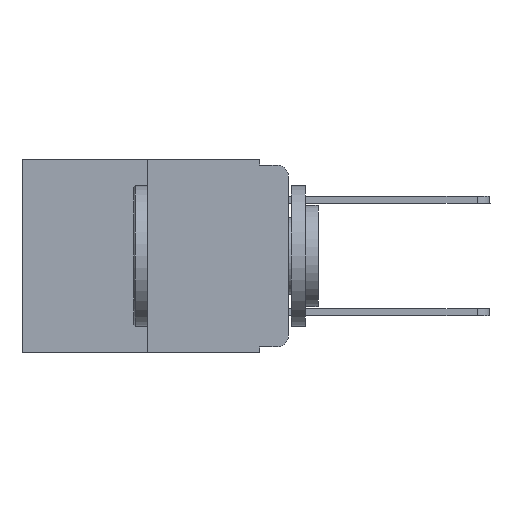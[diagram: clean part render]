
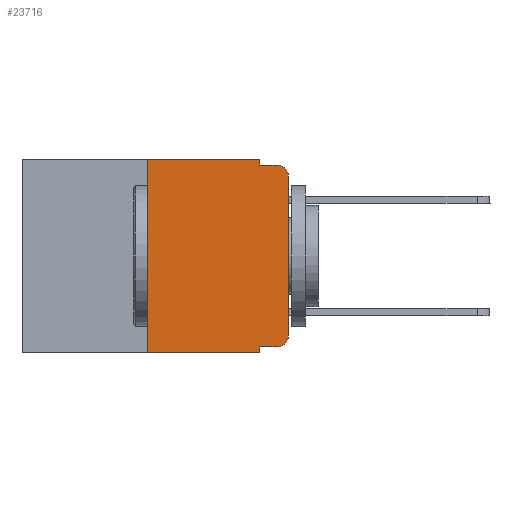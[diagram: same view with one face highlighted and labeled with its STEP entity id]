
A CAD part, left-side view. The second image highlights one B-rep face of the part: STEP entity #23716.
In plain terms, the highlighted planar face has unit normal (-1, 0, 0).
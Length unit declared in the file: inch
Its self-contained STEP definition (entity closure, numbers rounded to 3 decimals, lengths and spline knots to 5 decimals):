
#89 = DIRECTION ( 'NONE',  ( 0., 0., -1. ) ) ;
#220 = ORIENTED_EDGE ( 'NONE', *, *, #4690, .F. ) ;
#680 = CIRCLE ( 'NONE', #20054, 0.02 ) ;
#871 = VERTEX_POINT ( 'NONE', #3293 ) ;
#924 = AXIS2_PLACEMENT_3D ( 'NONE', #10022, #13965, #18078 ) ;
#1179 = ORIENTED_EDGE ( 'NONE', *, *, #4144, .T. ) ;
#1910 = ORIENTED_EDGE ( 'NONE', *, *, #21762, .T. ) ;
#2363 = VERTEX_POINT ( 'NONE', #22187 ) ;
#2385 = VECTOR ( 'NONE', #25052, 39.37008 ) ;
#2417 = CARTESIAN_POINT ( 'NONE',  ( 0., 0.051, -0.01 ) ) ;
#2907 = VERTEX_POINT ( 'NONE', #18002 ) ;
#3293 = CARTESIAN_POINT ( 'NONE',  ( 0., 0.051, -0.343 ) ) ;
#3735 = VECTOR ( 'NONE', #11981, 39.37008 ) ;
#3877 = VECTOR ( 'NONE', #17436, 39.37008 ) ;
#4144 = EDGE_CURVE ( 'NONE', #19177, #871, #5651, .T. ) ;
#4202 = VECTOR ( 'NONE', #18086, 39.37008 ) ;
#4552 = AXIS2_PLACEMENT_3D ( 'NONE', #26054, #11667, #21671 ) ;
#4689 = CARTESIAN_POINT ( 'NONE',  ( 0., 0.02, -0.333 ) ) ;
#4690 = EDGE_CURVE ( 'NONE', #19177, #2363, #14123, .T. ) ;
#4944 = CARTESIAN_POINT ( 'NONE',  ( 0., 0.051, 0. ) ) ;
#5037 = EDGE_CURVE ( 'NONE', #26030, #22423, #17229, .T. ) ;
#5310 = EDGE_CURVE ( 'NONE', #17140, #22423, #14396, .T. ) ;
#5575 = LINE ( 'NONE', #4944, #2385 ) ;
#5651 = LINE ( 'NONE', #24062, #3735 ) ;
#5678 = CARTESIAN_POINT ( 'NONE',  ( 0., 0.051, -0.333 ) ) ;
#5713 = EDGE_CURVE ( 'NONE', #19248, #26030, #5575, .T. ) ;
#6351 = FACE_OUTER_BOUND ( 'NONE', #14329, .T. ) ;
#6601 = ORIENTED_EDGE ( 'NONE', *, *, #5037, .F. ) ;
#8205 = CARTESIAN_POINT ( 'NONE',  ( 0., 0.02, -0.313 ) ) ;
#9725 = VECTOR ( 'NONE', #14063, 39.37008 ) ;
#9830 = DIRECTION ( 'NONE',  ( 0., 0., -1. ) ) ;
#9877 = CARTESIAN_POINT ( 'NONE',  ( 0., 0.25, 0. ) ) ;
#10022 = CARTESIAN_POINT ( 'NONE',  ( 0., 0.473, 0. ) ) ;
#10949 = ORIENTED_EDGE ( 'NONE', *, *, #15769, .T. ) ;
#11028 = VERTEX_POINT ( 'NONE', #4689 ) ;
#11283 = VECTOR ( 'NONE', #14648, 39.37008 ) ;
#11667 = DIRECTION ( 'NONE',  ( -1., 0., 0. ) ) ;
#11981 = DIRECTION ( 'NONE',  ( 0., -1., 0. ) ) ;
#12112 = PLANE ( 'NONE',  #924 ) ;
#12192 = CARTESIAN_POINT ( 'NONE',  ( 0., 0., -0.03 ) ) ;
#12262 = CARTESIAN_POINT ( 'NONE',  ( 0., 0.02, -0.01 ) ) ;
#12379 = CARTESIAN_POINT ( 'NONE',  ( 0., 0.051, -0.01 ) ) ;
#12767 = VERTEX_POINT ( 'NONE', #5678 ) ;
#13954 = EDGE_CURVE ( 'NONE', #2363, #19248, #23352, .T. ) ;
#13965 = DIRECTION ( 'NONE',  ( 1., 0., 0. ) ) ;
#14063 = DIRECTION ( 'NONE',  ( 0., -1., 0. ) ) ;
#14123 = LINE ( 'NONE', #9877, #25508 ) ;
#14143 = CARTESIAN_POINT ( 'NONE',  ( 0., 0.473, 0. ) ) ;
#14329 = EDGE_LOOP ( 'NONE', ( #1910, #15097, #6601, #15821, #15128, #220, #1179, #18156, #25757, #10949 ) ) ;
#14396 = CIRCLE ( 'NONE', #4552, 0.02 ) ;
#14648 = DIRECTION ( 'NONE',  ( 0., -1., 0. ) ) ;
#14969 = CARTESIAN_POINT ( 'NONE',  ( 0., 0.051, 0. ) ) ;
#15097 = ORIENTED_EDGE ( 'NONE', *, *, #5310, .T. ) ;
#15128 = ORIENTED_EDGE ( 'NONE', *, *, #13954, .F. ) ;
#15409 = CARTESIAN_POINT ( 'NONE',  ( 0., 0.051, -0.333 ) ) ;
#15769 = EDGE_CURVE ( 'NONE', #11028, #2907, #680, .T. ) ;
#15821 = ORIENTED_EDGE ( 'NONE', *, *, #5713, .F. ) ;
#16160 = LINE ( 'NONE', #20292, #4202 ) ;
#17140 = VERTEX_POINT ( 'NONE', #12192 ) ;
#17229 = LINE ( 'NONE', #2417, #11283 ) ;
#17436 = DIRECTION ( 'NONE',  ( 0., -1., 0. ) ) ;
#18002 = CARTESIAN_POINT ( 'NONE',  ( 0., 0., -0.313 ) ) ;
#18078 = DIRECTION ( 'NONE',  ( 0., 0., -1. ) ) ;
#18086 = DIRECTION ( 'NONE',  ( 0., 0., 1. ) ) ;
#18156 = ORIENTED_EDGE ( 'NONE', *, *, #20307, .F. ) ;
#18243 = VECTOR ( 'NONE', #9830, 39.37008 ) ;
#19177 = VERTEX_POINT ( 'NONE', #24707 ) ;
#19248 = VERTEX_POINT ( 'NONE', #14969 ) ;
#20054 = AXIS2_PLACEMENT_3D ( 'NONE', #8205, #20163, #89 ) ;
#20163 = DIRECTION ( 'NONE',  ( -1., 0., 0. ) ) ;
#20292 = CARTESIAN_POINT ( 'NONE',  ( 0., 0., 0. ) ) ;
#20307 = EDGE_CURVE ( 'NONE', #12767, #871, #20549, .T. ) ;
#20549 = LINE ( 'NONE', #24074, #18243 ) ;
#21671 = DIRECTION ( 'NONE',  ( 0., 0., -1. ) ) ;
#21762 = EDGE_CURVE ( 'NONE', #2907, #17140, #16160, .T. ) ;
#22126 = LINE ( 'NONE', #15409, #3877 ) ;
#22183 = EDGE_CURVE ( 'NONE', #12767, #11028, #22126, .T. ) ;
#22187 = CARTESIAN_POINT ( 'NONE',  ( 0., 0.25, 0. ) ) ;
#22423 = VERTEX_POINT ( 'NONE', #12262 ) ;
#23352 = LINE ( 'NONE', #14143, #9725 ) ;
#23716 = ADVANCED_FACE ( 'NONE', ( #6351 ), #12112, .F. ) ;
#24062 = CARTESIAN_POINT ( 'NONE',  ( 0., 0.473, -0.343 ) ) ;
#24074 = CARTESIAN_POINT ( 'NONE',  ( 0., 0.051, 0. ) ) ;
#24707 = CARTESIAN_POINT ( 'NONE',  ( 0., 0.25, -0.343 ) ) ;
#25052 = DIRECTION ( 'NONE',  ( 0., 0., -1. ) ) ;
#25508 = VECTOR ( 'NONE', #25557, 39.37008 ) ;
#25557 = DIRECTION ( 'NONE',  ( 0., 0., 1. ) ) ;
#25757 = ORIENTED_EDGE ( 'NONE', *, *, #22183, .T. ) ;
#26030 = VERTEX_POINT ( 'NONE', #12379 ) ;
#26054 = CARTESIAN_POINT ( 'NONE',  ( 0., 0.02, -0.03 ) ) ;
